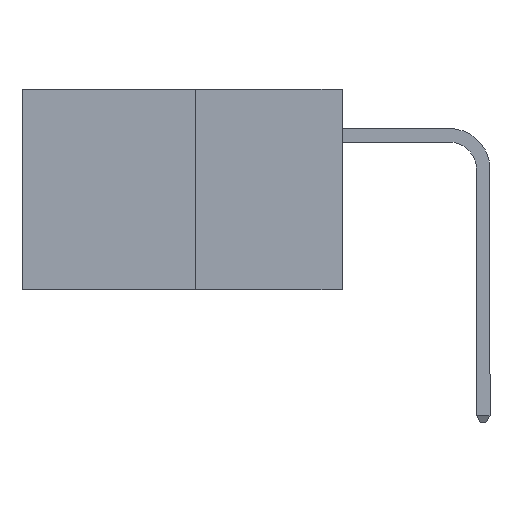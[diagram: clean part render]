
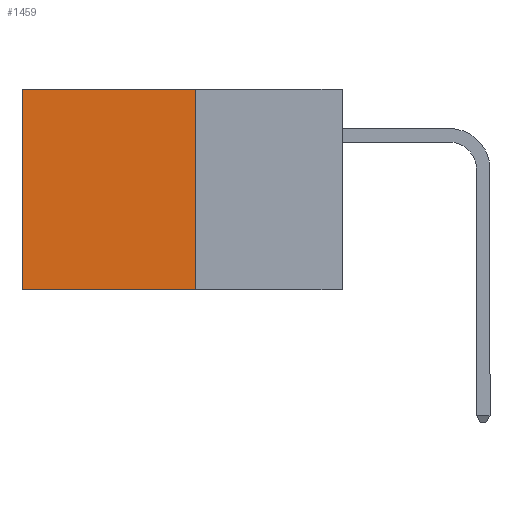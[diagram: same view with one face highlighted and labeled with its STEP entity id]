
A CAD part, left-side view. The second image highlights one B-rep face of the part: STEP entity #1459.
In plain terms, the highlighted planar face has unit normal (-1, 0, 0).
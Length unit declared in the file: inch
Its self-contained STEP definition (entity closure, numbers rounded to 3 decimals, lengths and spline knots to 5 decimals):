
#77 = CARTESIAN_POINT ( 'NONE',  ( 0.277, 0.27, -0.37 ) ) ;
#855 = VERTEX_POINT ( 'NONE', #8759 ) ;
#928 = ORIENTED_EDGE ( 'NONE', *, *, #3641, .F. ) ;
#971 = VECTOR ( 'NONE', #1647, 39.37008 ) ;
#1122 = LINE ( 'NONE', #77, #7222 ) ;
#1285 = LINE ( 'NONE', #6495, #7595 ) ;
#1444 = CARTESIAN_POINT ( 'NONE',  ( 0.277, 0.27, -0.37 ) ) ;
#1459 = ADVANCED_FACE ( 'NONE', ( #3616 ), #1748, .F. ) ;
#1647 = DIRECTION ( 'NONE',  ( 0., 1., 0. ) ) ;
#1748 = PLANE ( 'NONE',  #10573 ) ;
#1774 = CARTESIAN_POINT ( 'NONE',  ( 0.277, 0.27, 0. ) ) ;
#2766 = ORIENTED_EDGE ( 'NONE', *, *, #6092, .T. ) ;
#3256 = DIRECTION ( 'NONE',  ( 1., 0., 0. ) ) ;
#3616 = FACE_OUTER_BOUND ( 'NONE', #4848, .T. ) ;
#3641 = EDGE_CURVE ( 'NONE', #10239, #4947, #10409, .T. ) ;
#4029 = DIRECTION ( 'NONE',  ( 0., 0., -1. ) ) ;
#4711 = EDGE_CURVE ( 'NONE', #8823, #855, #1285, .T. ) ;
#4848 = EDGE_LOOP ( 'NONE', ( #8119, #8288, #928, #2766 ) ) ;
#4947 = VERTEX_POINT ( 'NONE', #10704 ) ;
#5744 = CARTESIAN_POINT ( 'NONE',  ( 0.277, 0.27, -0.37 ) ) ;
#5767 = DIRECTION ( 'NONE',  ( 0., 0., -1. ) ) ;
#6041 = DIRECTION ( 'NONE',  ( 0., 0., -1. ) ) ;
#6092 = EDGE_CURVE ( 'NONE', #10239, #8823, #9208, .T. ) ;
#6355 = EDGE_CURVE ( 'NONE', #4947, #855, #1122, .T. ) ;
#6495 = CARTESIAN_POINT ( 'NONE',  ( 0.277, 0.59, -0.37 ) ) ;
#7222 = VECTOR ( 'NONE', #10610, 39.37008 ) ;
#7590 = CARTESIAN_POINT ( 'NONE',  ( 0.277, 0.59, 0. ) ) ;
#7595 = VECTOR ( 'NONE', #6041, 39.37008 ) ;
#8119 = ORIENTED_EDGE ( 'NONE', *, *, #4711, .T. ) ;
#8288 = ORIENTED_EDGE ( 'NONE', *, *, #6355, .F. ) ;
#8673 = CARTESIAN_POINT ( 'NONE',  ( 0.277, 0.27, 0. ) ) ;
#8759 = CARTESIAN_POINT ( 'NONE',  ( 0.277, 0.59, -0.37 ) ) ;
#8823 = VERTEX_POINT ( 'NONE', #7590 ) ;
#9208 = LINE ( 'NONE', #1774, #971 ) ;
#10188 = VECTOR ( 'NONE', #5767, 39.37008 ) ;
#10239 = VERTEX_POINT ( 'NONE', #8673 ) ;
#10409 = LINE ( 'NONE', #5744, #10188 ) ;
#10573 = AXIS2_PLACEMENT_3D ( 'NONE', #1444, #3256, #4029 ) ;
#10610 = DIRECTION ( 'NONE',  ( 0., 1., 0. ) ) ;
#10704 = CARTESIAN_POINT ( 'NONE',  ( 0.277, 0.27, -0.37 ) ) ;
